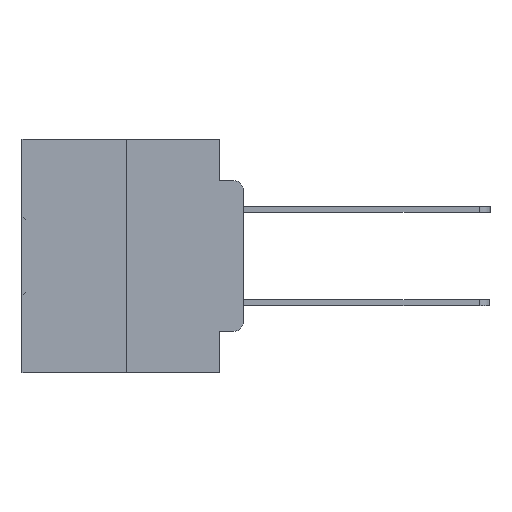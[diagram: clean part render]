
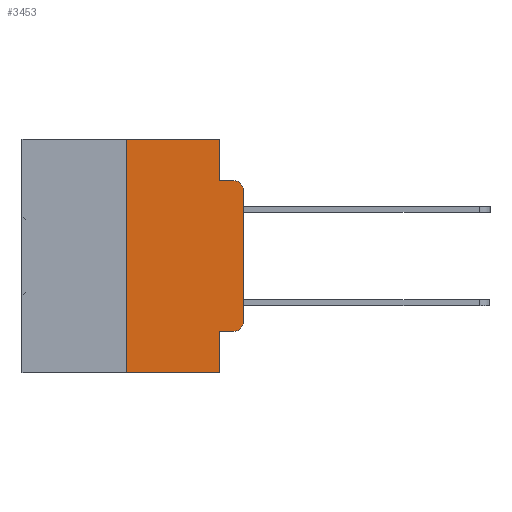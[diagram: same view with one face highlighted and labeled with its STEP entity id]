
A CAD part, left-side view. The second image highlights one B-rep face of the part: STEP entity #3453.
In plain terms, the highlighted planar face has unit normal (-1, 0, 0).
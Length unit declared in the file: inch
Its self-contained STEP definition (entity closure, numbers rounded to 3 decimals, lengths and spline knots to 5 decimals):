
#349 = AXIS2_PLACEMENT_3D ( 'NONE', #24249, #18561, #18521 ) ;
#643 = VECTOR ( 'NONE', #14550, 39.37008 ) ;
#966 = CARTESIAN_POINT ( 'NONE',  ( 0., 0.473, 0. ) ) ;
#1085 = CARTESIAN_POINT ( 'NONE',  ( 0., 0., -0.1085 ) ) ;
#1796 = LINE ( 'NONE', #18795, #29114 ) ;
#1832 = LINE ( 'NONE', #22367, #15616 ) ;
#3141 = EDGE_CURVE ( 'NONE', #13238, #15350, #12271, .T. ) ;
#3453 = ADVANCED_FACE ( 'NONE', ( #27486 ), #24589, .F. ) ;
#3761 = CARTESIAN_POINT ( 'NONE',  ( 0., 0.051, -0.0885 ) ) ;
#4968 = LINE ( 'NONE', #13983, #31359 ) ;
#5314 = EDGE_CURVE ( 'NONE', #18933, #13238, #1796, .T. ) ;
#5388 = DIRECTION ( 'NONE',  ( 0., 0., 1. ) ) ;
#6370 = CARTESIAN_POINT ( 'NONE',  ( 0., 0.051, -0.5 ) ) ;
#6655 = ORIENTED_EDGE ( 'NONE', *, *, #16800, .T. ) ;
#6720 = EDGE_CURVE ( 'NONE', #31246, #23363, #28249, .T. ) ;
#6747 = DIRECTION ( 'NONE',  ( -1., 0., 0. ) ) ;
#6858 = EDGE_CURVE ( 'NONE', #8238, #25585, #4968, .T. ) ;
#7887 = CARTESIAN_POINT ( 'NONE',  ( 0., 0.25, 0. ) ) ;
#8148 = EDGE_CURVE ( 'NONE', #29751, #25169, #21879, .T. ) ;
#8238 = VERTEX_POINT ( 'NONE', #31306 ) ;
#8394 = CARTESIAN_POINT ( 'NONE',  ( 0., 0.25, -0.5 ) ) ;
#9050 = CARTESIAN_POINT ( 'NONE',  ( 0., 0.25, 0. ) ) ;
#9108 = VECTOR ( 'NONE', #25485, 39.37008 ) ;
#10212 = VERTEX_POINT ( 'NONE', #1085 ) ;
#10747 = EDGE_CURVE ( 'NONE', #10212, #15350, #33014, .T. ) ;
#11252 = VECTOR ( 'NONE', #21659, 39.37008 ) ;
#11916 = CARTESIAN_POINT ( 'NONE',  ( 0., 0.051, -0.4115 ) ) ;
#11998 = CARTESIAN_POINT ( 'NONE',  ( 0., 0., -0.3915 ) ) ;
#12062 = LINE ( 'NONE', #966, #11252 ) ;
#12271 = LINE ( 'NONE', #12450, #16728 ) ;
#12450 = CARTESIAN_POINT ( 'NONE',  ( 0., 0.051, -0.0885 ) ) ;
#13238 = VERTEX_POINT ( 'NONE', #3761 ) ;
#13614 = CARTESIAN_POINT ( 'NONE',  ( 0., 0.02, -0.0885 ) ) ;
#13983 = CARTESIAN_POINT ( 'NONE',  ( 0., 0.051, 0. ) ) ;
#14550 = DIRECTION ( 'NONE',  ( 0., -1., 0. ) ) ;
#15051 = VECTOR ( 'NONE', #5388, 39.37008 ) ;
#15350 = VERTEX_POINT ( 'NONE', #13614 ) ;
#15616 = VECTOR ( 'NONE', #24902, 39.37008 ) ;
#16728 = VECTOR ( 'NONE', #28752, 39.37008 ) ;
#16800 = EDGE_CURVE ( 'NONE', #23363, #10212, #1832, .T. ) ;
#18521 = DIRECTION ( 'NONE',  ( 0., 0., -1. ) ) ;
#18561 = DIRECTION ( 'NONE',  ( 1., 0., 0. ) ) ;
#18795 = CARTESIAN_POINT ( 'NONE',  ( 0., 0.051, 0. ) ) ;
#18850 = ORIENTED_EDGE ( 'NONE', *, *, #6720, .T. ) ;
#18933 = VERTEX_POINT ( 'NONE', #23432 ) ;
#19476 = ORIENTED_EDGE ( 'NONE', *, *, #22991, .T. ) ;
#21212 = ORIENTED_EDGE ( 'NONE', *, *, #5314, .F. ) ;
#21583 = DIRECTION ( 'NONE',  ( 0., 0., -1. ) ) ;
#21659 = DIRECTION ( 'NONE',  ( 0., -1., 0. ) ) ;
#21879 = LINE ( 'NONE', #7887, #15051 ) ;
#21970 = EDGE_LOOP ( 'NONE', ( #6655, #30370, #32680, #21212, #22799, #22389, #19476, #24567, #32253, #18850 ) ) ;
#22227 = CARTESIAN_POINT ( 'NONE',  ( 0., 0.02, -0.1085 ) ) ;
#22367 = CARTESIAN_POINT ( 'NONE',  ( 0., 0., 0. ) ) ;
#22389 = ORIENTED_EDGE ( 'NONE', *, *, #8148, .F. ) ;
#22799 = ORIENTED_EDGE ( 'NONE', *, *, #31536, .F. ) ;
#22991 = EDGE_CURVE ( 'NONE', #29751, #25585, #24399, .T. ) ;
#23363 = VERTEX_POINT ( 'NONE', #11998 ) ;
#23432 = CARTESIAN_POINT ( 'NONE',  ( 0., 0.051, 0. ) ) ;
#24249 = CARTESIAN_POINT ( 'NONE',  ( 0., 0.473, 0. ) ) ;
#24399 = LINE ( 'NONE', #32748, #9108 ) ;
#24567 = ORIENTED_EDGE ( 'NONE', *, *, #6858, .F. ) ;
#24589 = PLANE ( 'NONE',  #349 ) ;
#24765 = DIRECTION ( 'NONE',  ( 0., 0., -1. ) ) ;
#24902 = DIRECTION ( 'NONE',  ( 0., 0., 1. ) ) ;
#25169 = VERTEX_POINT ( 'NONE', #9050 ) ;
#25297 = DIRECTION ( 'NONE',  ( 0., 0., -1. ) ) ;
#25368 = DIRECTION ( 'NONE',  ( -1., 0., 0. ) ) ;
#25485 = DIRECTION ( 'NONE',  ( 0., -1., 0. ) ) ;
#25521 = CARTESIAN_POINT ( 'NONE',  ( 0., 0.02, -0.3915 ) ) ;
#25585 = VERTEX_POINT ( 'NONE', #6370 ) ;
#27252 = LINE ( 'NONE', #11916, #643 ) ;
#27486 = FACE_OUTER_BOUND ( 'NONE', #21970, .T. ) ;
#27989 = CARTESIAN_POINT ( 'NONE',  ( 0., 0.02, -0.4115 ) ) ;
#28249 = CIRCLE ( 'NONE', #32151, 0.02 ) ;
#28752 = DIRECTION ( 'NONE',  ( 0., -1., 0. ) ) ;
#28911 = DIRECTION ( 'NONE',  ( 0., 0., -1. ) ) ;
#29114 = VECTOR ( 'NONE', #28911, 39.37008 ) ;
#29131 = AXIS2_PLACEMENT_3D ( 'NONE', #22227, #6747, #24765 ) ;
#29751 = VERTEX_POINT ( 'NONE', #8394 ) ;
#30370 = ORIENTED_EDGE ( 'NONE', *, *, #10747, .T. ) ;
#31246 = VERTEX_POINT ( 'NONE', #27989 ) ;
#31306 = CARTESIAN_POINT ( 'NONE',  ( 0., 0.051, -0.4115 ) ) ;
#31359 = VECTOR ( 'NONE', #21583, 39.37008 ) ;
#31536 = EDGE_CURVE ( 'NONE', #25169, #18933, #12062, .T. ) ;
#32151 = AXIS2_PLACEMENT_3D ( 'NONE', #25521, #25368, #25297 ) ;
#32253 = ORIENTED_EDGE ( 'NONE', *, *, #32312, .T. ) ;
#32312 = EDGE_CURVE ( 'NONE', #8238, #31246, #27252, .T. ) ;
#32680 = ORIENTED_EDGE ( 'NONE', *, *, #3141, .F. ) ;
#32748 = CARTESIAN_POINT ( 'NONE',  ( 0., 0.473, -0.5 ) ) ;
#33014 = CIRCLE ( 'NONE', #29131, 0.02 ) ;
